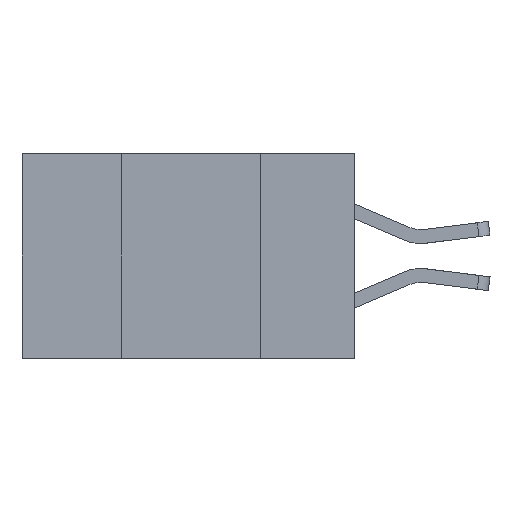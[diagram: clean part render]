
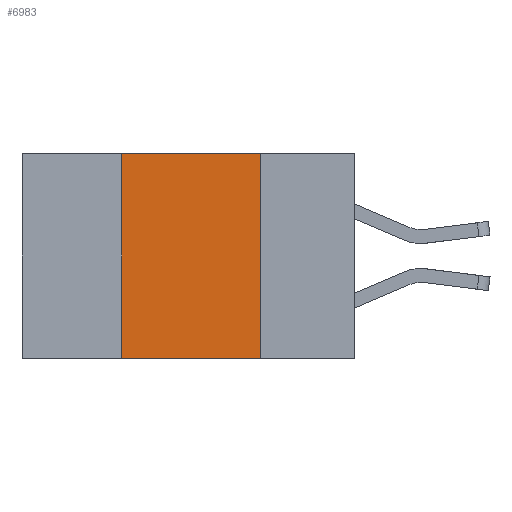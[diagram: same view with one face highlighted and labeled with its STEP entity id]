
A CAD part, left-side view. The second image highlights one B-rep face of the part: STEP entity #6983.
In plain terms, the highlighted planar face has unit normal (-1, 0, 0).
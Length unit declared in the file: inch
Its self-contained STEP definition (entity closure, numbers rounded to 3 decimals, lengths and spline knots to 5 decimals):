
#415 = ORIENTED_EDGE ( 'NONE', *, *, #6704, .T. ) ;
#437 = VERTEX_POINT ( 'NONE', #5186 ) ;
#2044 = EDGE_CURVE ( 'NONE', #437, #7040, #5030, .T. ) ;
#2496 = EDGE_CURVE ( 'NONE', #4153, #8829, #6925, .T. ) ;
#3093 = CARTESIAN_POINT ( 'NONE',  ( 0., 0.6, -0.37 ) ) ;
#3860 = CARTESIAN_POINT ( 'NONE',  ( 0., 0.17, -0.37 ) ) ;
#3964 = DIRECTION ( 'NONE',  ( 0., 0., -1. ) ) ;
#4153 = VERTEX_POINT ( 'NONE', #4583 ) ;
#4335 = DIRECTION ( 'NONE',  ( 0., 0., -1. ) ) ;
#4505 = CARTESIAN_POINT ( 'NONE',  ( 0., 0.42, 0. ) ) ;
#4583 = CARTESIAN_POINT ( 'NONE',  ( 0., 0.42, -0.37 ) ) ;
#4639 = PLANE ( 'NONE',  #8189 ) ;
#4642 = VECTOR ( 'NONE', #8113, 39.37008 ) ;
#4861 = ORIENTED_EDGE ( 'NONE', *, *, #2496, .F. ) ;
#4872 = VECTOR ( 'NONE', #8666, 39.37008 ) ;
#5030 = LINE ( 'NONE', #6154, #6676 ) ;
#5176 = EDGE_LOOP ( 'NONE', ( #8079, #5536, #4861, #415 ) ) ;
#5186 = CARTESIAN_POINT ( 'NONE',  ( 0., 0.17, 0. ) ) ;
#5536 = ORIENTED_EDGE ( 'NONE', *, *, #7570, .F. ) ;
#6154 = CARTESIAN_POINT ( 'NONE',  ( 0., 0.17, 0. ) ) ;
#6306 = CARTESIAN_POINT ( 'NONE',  ( 0., 0.42, 0. ) ) ;
#6489 = LINE ( 'NONE', #7597, #7851 ) ;
#6643 = LINE ( 'NONE', #3093, #4872 ) ;
#6676 = VECTOR ( 'NONE', #4335, 39.37008 ) ;
#6704 = EDGE_CURVE ( 'NONE', #4153, #7040, #6643, .T. ) ;
#6925 = LINE ( 'NONE', #6306, #4642 ) ;
#6983 = ADVANCED_FACE ( 'NONE', ( #7376 ), #4639, .F. ) ;
#7040 = VERTEX_POINT ( 'NONE', #3860 ) ;
#7072 = DIRECTION ( 'NONE',  ( 1., 0., 0. ) ) ;
#7376 = FACE_OUTER_BOUND ( 'NONE', #5176, .T. ) ;
#7570 = EDGE_CURVE ( 'NONE', #8829, #437, #6489, .T. ) ;
#7597 = CARTESIAN_POINT ( 'NONE',  ( 0., 0.6, 0. ) ) ;
#7626 = DIRECTION ( 'NONE',  ( 0., -1., 0. ) ) ;
#7851 = VECTOR ( 'NONE', #7626, 39.37008 ) ;
#8079 = ORIENTED_EDGE ( 'NONE', *, *, #2044, .F. ) ;
#8113 = DIRECTION ( 'NONE',  ( 0., 0., 1. ) ) ;
#8189 = AXIS2_PLACEMENT_3D ( 'NONE', #10261, #7072, #3964 ) ;
#8666 = DIRECTION ( 'NONE',  ( 0., -1., 0. ) ) ;
#8829 = VERTEX_POINT ( 'NONE', #4505 ) ;
#10261 = CARTESIAN_POINT ( 'NONE',  ( 0., 0.6, 0. ) ) ;
